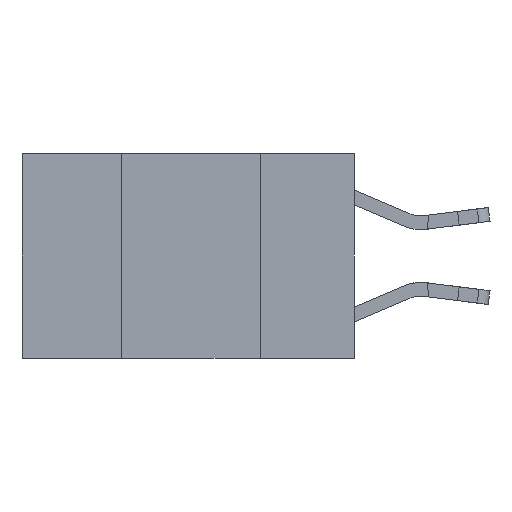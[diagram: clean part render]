
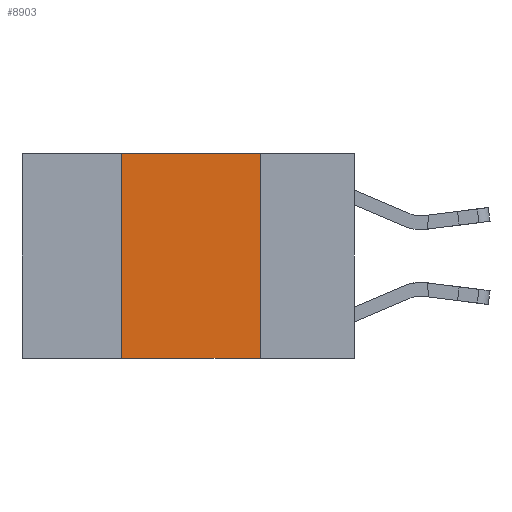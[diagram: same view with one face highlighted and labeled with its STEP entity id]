
A CAD part, left-side view. The second image highlights one B-rep face of the part: STEP entity #8903.
In plain terms, the highlighted planar face has unit normal (-1, 0, 0).
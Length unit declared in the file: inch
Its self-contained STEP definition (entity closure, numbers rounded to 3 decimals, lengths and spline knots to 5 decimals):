
#681 = VERTEX_POINT ( 'NONE', #18164 ) ;
#743 = DIRECTION ( 'NONE',  ( 0., 0., 1. ) ) ;
#861 = DIRECTION ( 'NONE',  ( 0., 0., -1. ) ) ;
#1954 = FACE_OUTER_BOUND ( 'NONE', #2478, .T. ) ;
#2478 = EDGE_LOOP ( 'NONE', ( #18322, #6393, #6445, #10258 ) ) ;
#2775 = CARTESIAN_POINT ( 'NONE',  ( 0., 0.42, 0. ) ) ;
#3735 = CARTESIAN_POINT ( 'NONE',  ( 0., 0.42, -0.37 ) ) ;
#4058 = EDGE_CURVE ( 'NONE', #8280, #6208, #11905, .T. ) ;
#5248 = EDGE_CURVE ( 'NONE', #6208, #681, #14376, .T. ) ;
#5448 = CARTESIAN_POINT ( 'NONE',  ( 0., 0.17, 0. ) ) ;
#5690 = CARTESIAN_POINT ( 'NONE',  ( 0., 0.6, 0. ) ) ;
#6208 = VERTEX_POINT ( 'NONE', #5448 ) ;
#6210 = EDGE_CURVE ( 'NONE', #18368, #681, #14625, .T. ) ;
#6318 = VECTOR ( 'NONE', #11707, 39.37008 ) ;
#6393 = ORIENTED_EDGE ( 'NONE', *, *, #4058, .F. ) ;
#6445 = ORIENTED_EDGE ( 'NONE', *, *, #15734, .F. ) ;
#7040 = CARTESIAN_POINT ( 'NONE',  ( 0., 0.6, -0.37 ) ) ;
#7548 = VECTOR ( 'NONE', #743, 39.37008 ) ;
#8280 = VERTEX_POINT ( 'NONE', #2775 ) ;
#8903 = ADVANCED_FACE ( 'NONE', ( #1954 ), #9163, .F. ) ;
#9163 = PLANE ( 'NONE',  #19380 ) ;
#9704 = LINE ( 'NONE', #14253, #7548 ) ;
#9844 = VECTOR ( 'NONE', #861, 39.37008 ) ;
#10258 = ORIENTED_EDGE ( 'NONE', *, *, #6210, .T. ) ;
#10314 = VECTOR ( 'NONE', #13037, 39.37008 ) ;
#11707 = DIRECTION ( 'NONE',  ( 0., -1., 0. ) ) ;
#11905 = LINE ( 'NONE', #5690, #6318 ) ;
#13037 = DIRECTION ( 'NONE',  ( 0., -1., 0. ) ) ;
#13697 = DIRECTION ( 'NONE',  ( 1., 0., 0. ) ) ;
#14253 = CARTESIAN_POINT ( 'NONE',  ( 0., 0.42, 0. ) ) ;
#14376 = LINE ( 'NONE', #17453, #9844 ) ;
#14625 = LINE ( 'NONE', #7040, #10314 ) ;
#15206 = CARTESIAN_POINT ( 'NONE',  ( 0., 0.6, 0. ) ) ;
#15734 = EDGE_CURVE ( 'NONE', #18368, #8280, #9704, .T. ) ;
#16581 = DIRECTION ( 'NONE',  ( 0., 0., -1. ) ) ;
#17453 = CARTESIAN_POINT ( 'NONE',  ( 0., 0.17, 0. ) ) ;
#18164 = CARTESIAN_POINT ( 'NONE',  ( 0., 0.17, -0.37 ) ) ;
#18322 = ORIENTED_EDGE ( 'NONE', *, *, #5248, .F. ) ;
#18368 = VERTEX_POINT ( 'NONE', #3735 ) ;
#19380 = AXIS2_PLACEMENT_3D ( 'NONE', #15206, #13697, #16581 ) ;
